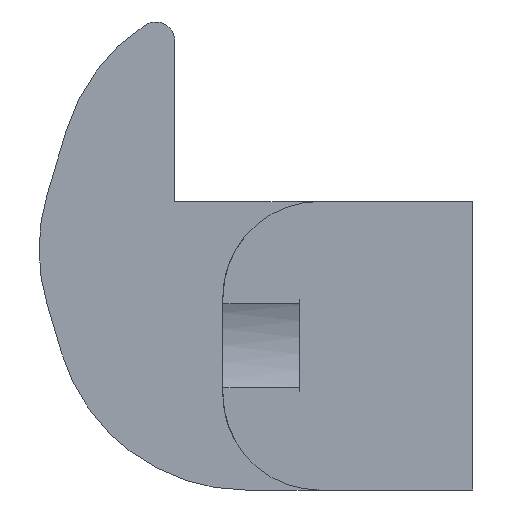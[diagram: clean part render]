
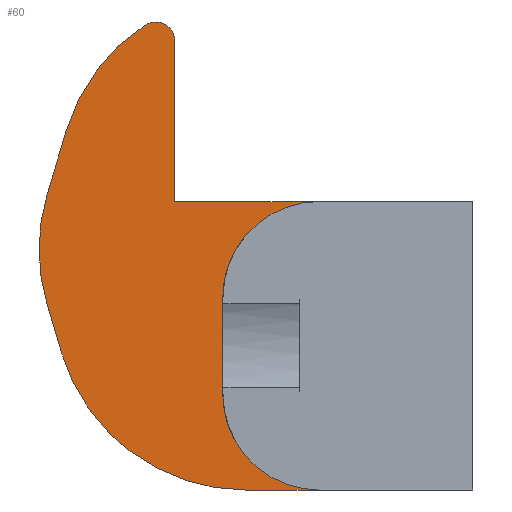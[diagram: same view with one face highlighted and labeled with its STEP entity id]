
A CAD part, left-side view. The second image highlights one B-rep face of the part: STEP entity #60.
In plain terms, the highlighted planar face has unit normal (-1, 0, 0).
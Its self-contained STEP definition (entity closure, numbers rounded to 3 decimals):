
#4 = CARTESIAN_POINT ( 'NONE',  ( -3.75, 2.024, 12.085 ) ) ;
#60 = ADVANCED_FACE ( 'NONE', ( #1422 ), #269, .T. ) ;
#75 = CARTESIAN_POINT ( 'NONE',  ( -3.75, 0., 7.5 ) ) ;
#78 = VERTEX_POINT ( 'NONE', #676 ) ;
#79 = DIRECTION ( 'NONE',  ( 0., 0.287, -0.958 ) ) ;
#84 = CARTESIAN_POINT ( 'NONE',  ( -3.75, 0., 0. ) ) ;
#102 = DIRECTION ( 'NONE',  ( 0., 1., 0. ) ) ;
#145 = ORIENTED_EDGE ( 'NONE', *, *, #1208, .T. ) ;
#160 = CARTESIAN_POINT ( 'NONE',  ( -3.75, 1.75, 11.667 ) ) ;
#161 = ORIENTED_EDGE ( 'NONE', *, *, #1233, .T. ) ;
#189 = DIRECTION ( 'NONE',  ( -1., 0., 0. ) ) ;
#195 = DIRECTION ( 'NONE',  ( 0., 0., 1. ) ) ;
#200 = DIRECTION ( 'NONE',  ( -1., 0., 0. ) ) ;
#205 = CARTESIAN_POINT ( 'NONE',  ( -3.75, 4.073, 9.339 ) ) ;
#246 = DIRECTION ( 'NONE',  ( 0., 0., 1. ) ) ;
#251 = CARTESIAN_POINT ( 'NONE',  ( -3.75, -2.5, 2.5 ) ) ;
#267 = CARTESIAN_POINT ( 'NONE',  ( -3.75, 1.25, 12.5 ) ) ;
#269 = PLANE ( 'NONE',  #903 ) ;
#275 = CARTESIAN_POINT ( 'NONE',  ( -3.75, 1.75, 11.667 ) ) ;
#285 = VERTEX_POINT ( 'NONE', #205 ) ;
#319 = ORIENTED_EDGE ( 'NONE', *, *, #1083, .F. ) ;
#342 = VECTOR ( 'NONE', #527, 1000. ) ;
#343 = CIRCLE ( 'NONE', #592, 2.5 ) ;
#358 = LINE ( 'NONE', #84, #342 ) ;
#360 = VECTOR ( 'NONE', #901, 1000. ) ;
#362 = LINE ( 'NONE', #1298, #360 ) ;
#365 = DIRECTION ( 'NONE',  ( 0., 0., 1. ) ) ;
#366 = ORIENTED_EDGE ( 'NONE', *, *, #1220, .T. ) ;
#367 = VECTOR ( 'NONE', #79, 1000. ) ;
#370 = LINE ( 'NONE', #893, #367 ) ;
#373 = CIRCLE ( 'NONE', #602, 5. ) ;
#377 = CIRCLE ( 'NONE', #598, 2.5 ) ;
#380 = VERTEX_POINT ( 'NONE', #879 ) ;
#386 = DIRECTION ( 'NONE',  ( 0., 0., 1. ) ) ;
#391 = CIRCLE ( 'NONE', #601, 5. ) ;
#394 = DIRECTION ( 'NONE',  ( -1., 0., 0. ) ) ;
#396 = VECTOR ( 'NONE', #1396, 1000. ) ;
#398 = CIRCLE ( 'NONE', #606, 5. ) ;
#411 = CARTESIAN_POINT ( 'NONE',  ( -3.75, 0., 3.75 ) ) ;
#415 = CARTESIAN_POINT ( 'NONE',  ( -3.75, 0., 7.5 ) ) ;
#417 = CIRCLE ( 'NONE', #607, 0.5 ) ;
#438 = LINE ( 'NONE', #267, #396 ) ;
#448 = CARTESIAN_POINT ( 'NONE',  ( -3.75, 0., 2.5 ) ) ;
#466 = CARTESIAN_POINT ( 'NONE',  ( -3.75, 4.194, 3.563 ) ) ;
#525 = ORIENTED_EDGE ( 'NONE', *, *, #1230, .T. ) ;
#527 = DIRECTION ( 'NONE',  ( 0., 1., 0. ) ) ;
#533 = CARTESIAN_POINT ( 'NONE',  ( -3.75, 4.569, 7.687 ) ) ;
#592 = AXIS2_PLACEMENT_3D ( 'NONE', #1380, #612, #1474 ) ;
#598 = AXIS2_PLACEMENT_3D ( 'NONE', #251, #1142, #365 ) ;
#600 = VERTEX_POINT ( 'NONE', #448 ) ;
#601 = AXIS2_PLACEMENT_3D ( 'NONE', #907, #189, #1043 ) ;
#602 = AXIS2_PLACEMENT_3D ( 'NONE', #1181, #394, #1303 ) ;
#606 = AXIS2_PLACEMENT_3D ( 'NONE', #1401, #644, #1497 ) ;
#607 = AXIS2_PLACEMENT_3D ( 'NONE', #275, #1171, #386 ) ;
#612 = DIRECTION ( 'NONE',  ( 1., 0., 0. ) ) ;
#644 = DIRECTION ( 'NONE',  ( -1., 0., 0. ) ) ;
#676 = CARTESIAN_POINT ( 'NONE',  ( -3.75, 0., 5. ) ) ;
#699 = VECTOR ( 'NONE', #792, 1000. ) ;
#713 = VERTEX_POINT ( 'NONE', #4 ) ;
#715 = VECTOR ( 'NONE', #1306, 1000. ) ;
#716 = LINE ( 'NONE', #1319, #699 ) ;
#720 = ORIENTED_EDGE ( 'NONE', *, *, #1227, .T. ) ;
#733 = LINE ( 'NONE', #75, #715 ) ;
#758 = AXIS2_PLACEMENT_3D ( 'NONE', #160, #998, #246 ) ;
#788 = CARTESIAN_POINT ( 'NONE',  ( -3.75, 0., 7.5 ) ) ;
#792 = DIRECTION ( 'NONE',  ( 0., 0., -1. ) ) ;
#852 = ORIENTED_EDGE ( 'NONE', *, *, #1217, .T. ) ;
#863 = ORIENTED_EDGE ( 'NONE', *, *, #1205, .F. ) ;
#879 = CARTESIAN_POINT ( 'NONE',  ( -3.75, 4.569, 4.813 ) ) ;
#893 = CARTESIAN_POINT ( 'NONE',  ( -3.75, 4.243, 8.773 ) ) ;
#901 = DIRECTION ( 'NONE',  ( 0., -0.287, -0.958 ) ) ;
#903 = AXIS2_PLACEMENT_3D ( 'NONE', #415, #200, #195 ) ;
#907 = CARTESIAN_POINT ( 'NONE',  ( -3.75, -0.595, 5. ) ) ;
#921 = VERTEX_POINT ( 'NONE', #1471 ) ;
#922 = EDGE_CURVE ( 'NONE', #1268, #1051, #1198, .T. ) ;
#947 = VERTEX_POINT ( 'NONE', #533 ) ;
#952 = VERTEX_POINT ( 'NONE', #466 ) ;
#955 = LINE ( 'NONE', #788, #956 ) ;
#956 = VECTOR ( 'NONE', #102, 1000. ) ;
#962 = ORIENTED_EDGE ( 'NONE', *, *, #922, .T. ) ;
#966 = ORIENTED_EDGE ( 'NONE', *, *, #1079, .F. ) ;
#989 = EDGE_CURVE ( 'NONE', #1375, #1378, #955, .T. ) ;
#998 = DIRECTION ( 'NONE',  ( -1., 0., 0. ) ) ;
#1036 = CARTESIAN_POINT ( 'NONE',  ( -3.75, -2.5, 7.5 ) ) ;
#1043 = DIRECTION ( 'NONE',  ( 0., 0., 1. ) ) ;
#1051 = VERTEX_POINT ( 'NONE', #1301 ) ;
#1079 = EDGE_CURVE ( 'NONE', #78, #1513, #733, .T. ) ;
#1083 = EDGE_CURVE ( 'NONE', #1513, #600, #716, .T. ) ;
#1142 = DIRECTION ( 'NONE',  ( 1., 0., 0. ) ) ;
#1156 = ORIENTED_EDGE ( 'NONE', *, *, #1229, .F. ) ;
#1171 = DIRECTION ( 'NONE',  ( -1., 0., 0. ) ) ;
#1181 = CARTESIAN_POINT ( 'NONE',  ( -3.75, -0.22, 6.25 ) ) ;
#1182 = CARTESIAN_POINT ( 'NONE',  ( -3.75, 1.25, 7.5 ) ) ;
#1198 = CIRCLE ( 'NONE', #758, 0.5 ) ;
#1205 = EDGE_CURVE ( 'NONE', #1268, #1378, #438, .T. ) ;
#1208 = EDGE_CURVE ( 'NONE', #1051, #713, #417, .T. ) ;
#1214 = EDGE_CURVE ( 'NONE', #713, #285, #398, .T. ) ;
#1217 = EDGE_CURVE ( 'NONE', #285, #947, #370, .T. ) ;
#1220 = EDGE_CURVE ( 'NONE', #947, #380, #373, .T. ) ;
#1222 = EDGE_CURVE ( 'NONE', #380, #952, #362, .T. ) ;
#1227 = EDGE_CURVE ( 'NONE', #952, #1261, #391, .T. ) ;
#1229 = EDGE_CURVE ( 'NONE', #921, #1261, #358, .T. ) ;
#1230 = EDGE_CURVE ( 'NONE', #921, #600, #377, .T. ) ;
#1233 = EDGE_CURVE ( 'NONE', #78, #1375, #343, .T. ) ;
#1261 = VERTEX_POINT ( 'NONE', #1386 ) ;
#1268 = VERTEX_POINT ( 'NONE', #1285 ) ;
#1278 = EDGE_LOOP ( 'NONE', ( #863, #962, #145, #1441, #852, #366, #1429, #720, #1156, #525, #319, #966, #161, #1302 ) ) ;
#1285 = CARTESIAN_POINT ( 'NONE',  ( -3.75, 1.25, 11.667 ) ) ;
#1298 = CARTESIAN_POINT ( 'NONE',  ( -3.75, 4.931, 6.021 ) ) ;
#1301 = CARTESIAN_POINT ( 'NONE',  ( -3.75, 1.75, 12.167 ) ) ;
#1302 = ORIENTED_EDGE ( 'NONE', *, *, #989, .T. ) ;
#1303 = DIRECTION ( 'NONE',  ( 0., 0., 1. ) ) ;
#1306 = DIRECTION ( 'NONE',  ( 0., 0., -1. ) ) ;
#1319 = CARTESIAN_POINT ( 'NONE',  ( -3.75, 0., 7.5 ) ) ;
#1375 = VERTEX_POINT ( 'NONE', #1036 ) ;
#1378 = VERTEX_POINT ( 'NONE', #1182 ) ;
#1380 = CARTESIAN_POINT ( 'NONE',  ( -3.75, -2.5, 5. ) ) ;
#1386 = CARTESIAN_POINT ( 'NONE',  ( -3.75, -0.595, 0. ) ) ;
#1396 = DIRECTION ( 'NONE',  ( 0., 0., -1. ) ) ;
#1401 = CARTESIAN_POINT ( 'NONE',  ( -3.75, -0.716, 7.903 ) ) ;
#1422 = FACE_OUTER_BOUND ( 'NONE', #1278, .T. ) ;
#1429 = ORIENTED_EDGE ( 'NONE', *, *, #1222, .T. ) ;
#1441 = ORIENTED_EDGE ( 'NONE', *, *, #1214, .T. ) ;
#1471 = CARTESIAN_POINT ( 'NONE',  ( -3.75, -2.5, 0. ) ) ;
#1474 = DIRECTION ( 'NONE',  ( 0., 0., 1. ) ) ;
#1497 = DIRECTION ( 'NONE',  ( 0., 0., 1. ) ) ;
#1513 = VERTEX_POINT ( 'NONE', #411 ) ;
